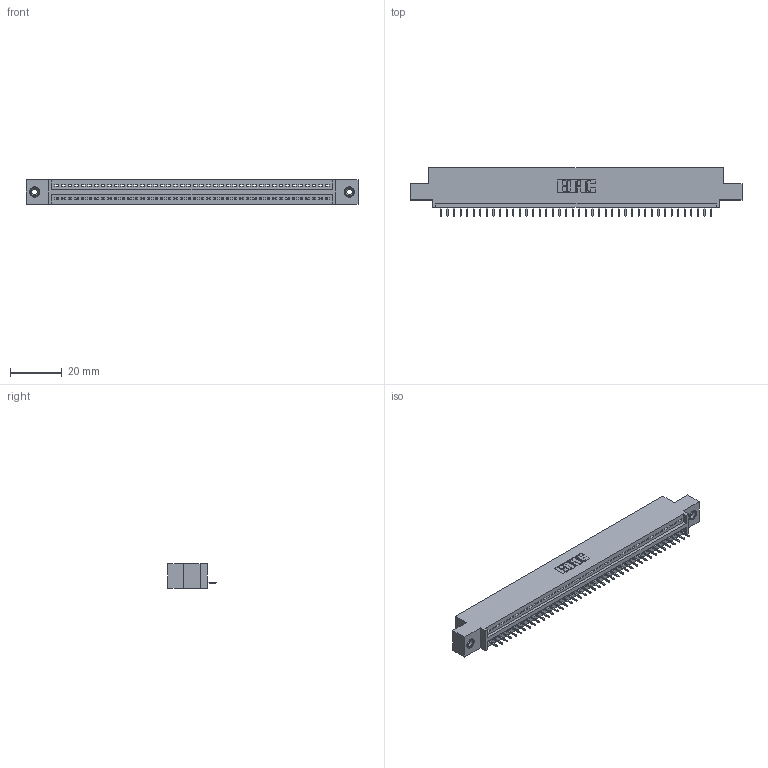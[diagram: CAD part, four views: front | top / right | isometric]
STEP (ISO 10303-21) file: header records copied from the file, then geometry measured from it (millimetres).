
FILE_DESCRIPTION (( 'STEP AP203' ), '1' );
FILE_NAME ('895-042-525-408.STEP', '2020-09-27T01:42:49', ( '' ), ( '' ), 'SwSTEP 2.0', 'SolidWorks 2020', '' );
FILE_SCHEMA (( 'CONFIG_CONTROL_DESIGN' ));
Length unit declared in the file: inch
Products named in the file (4): 895-042-525-408; 345-250-001_345-250-003-102; 345-292-001_345-293-125; 845 Part_0.110 Offset - 0.156 Dia-TI
Assembly tree (45 placements, depth 2):
  895-042-525-408
    845 Part_0.110 Offset - 0.156 Dia-TI
    345-292-001_345-293-125  x42
    345-250-001_345-250-003-102  x2
Bounding box: 127.89 x 18.72 x 9.4 mm (x, y, z)
Volume: 11895.7 mm3; surface area: 15337.4 mm2
Topology: 45 solids, 45 shells, 2794 faces, 8049 edges, 5190 vertices
Faces by surface type: plane 2048, cylinder 730, cone 12, torus 4
Entity records: 33002 total; most frequent: CARTESIAN_POINT 5697, ORIENTED_EDGE 5666, DIRECTION 5003, EDGE_CURVE 2833, VECTOR 2517, LINE 2517, VERTEX_POINT 1880, AXIS2_PLACEMENT_3D 1243
